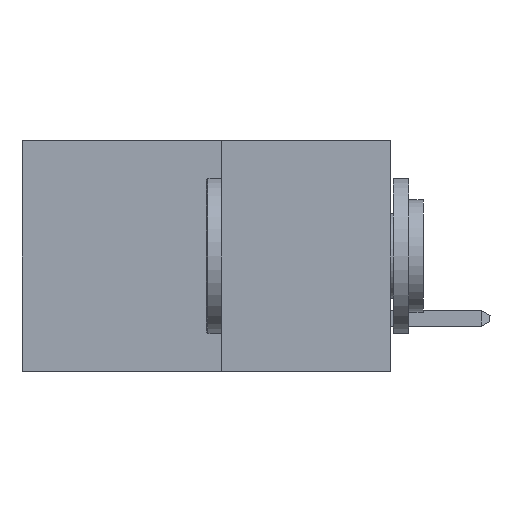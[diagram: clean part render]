
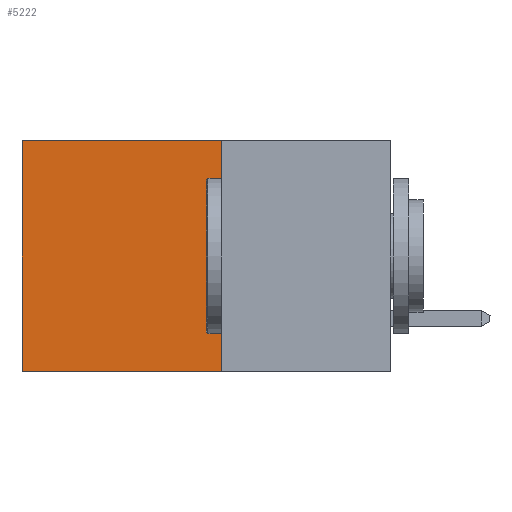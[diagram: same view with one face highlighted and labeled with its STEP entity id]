
A CAD part, left-side view. The second image highlights one B-rep face of the part: STEP entity #5222.
In plain terms, the highlighted planar face has unit normal (-1, 0, 0).
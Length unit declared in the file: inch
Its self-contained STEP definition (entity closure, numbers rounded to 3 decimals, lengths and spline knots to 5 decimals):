
#115 = ORIENTED_EDGE ( 'NONE', *, *, #12613, .F. ) ;
#355 = VERTEX_POINT ( 'NONE', #15876 ) ;
#586 = EDGE_CURVE ( 'NONE', #9196, #2411, #7843, .T. ) ;
#703 = VECTOR ( 'NONE', #13548, 39.37008 ) ;
#725 = CARTESIAN_POINT ( 'NONE',  ( 0.277, 0.27, -0.37 ) ) ;
#857 = DIRECTION ( 'NONE',  ( 0., 0., -1. ) ) ;
#893 = EDGE_CURVE ( 'NONE', #2411, #5199, #7447, .T. ) ;
#1137 = VECTOR ( 'NONE', #9937, 39.37008 ) ;
#1977 = LINE ( 'NONE', #725, #2400 ) ;
#2245 = FACE_OUTER_BOUND ( 'NONE', #8355, .T. ) ;
#2400 = VECTOR ( 'NONE', #857, 39.37008 ) ;
#2411 = VERTEX_POINT ( 'NONE', #9262 ) ;
#4274 = AXIS2_PLACEMENT_3D ( 'NONE', #14201, #14146, #14125 ) ;
#4590 = VECTOR ( 'NONE', #15267, 39.37008 ) ;
#5199 = VERTEX_POINT ( 'NONE', #14320 ) ;
#5222 = ADVANCED_FACE ( 'NONE', ( #2245 ), #14271, .F. ) ;
#6956 = EDGE_CURVE ( 'NONE', #9196, #355, #1977, .T. ) ;
#7447 = LINE ( 'NONE', #8086, #703 ) ;
#7487 = ORIENTED_EDGE ( 'NONE', *, *, #586, .T. ) ;
#7843 = LINE ( 'NONE', #13983, #1137 ) ;
#8086 = CARTESIAN_POINT ( 'NONE',  ( 0.277, 0.59, -0.37 ) ) ;
#8355 = EDGE_LOOP ( 'NONE', ( #14145, #115, #10643, #7487 ) ) ;
#9196 = VERTEX_POINT ( 'NONE', #12678 ) ;
#9262 = CARTESIAN_POINT ( 'NONE',  ( 0.277, 0.59, 0. ) ) ;
#9937 = DIRECTION ( 'NONE',  ( 0., 1., 0. ) ) ;
#10643 = ORIENTED_EDGE ( 'NONE', *, *, #6956, .F. ) ;
#12613 = EDGE_CURVE ( 'NONE', #355, #5199, #13869, .T. ) ;
#12678 = CARTESIAN_POINT ( 'NONE',  ( 0.277, 0.27, 0. ) ) ;
#12921 = CARTESIAN_POINT ( 'NONE',  ( 0.277, 0.27, -0.37 ) ) ;
#13548 = DIRECTION ( 'NONE',  ( 0., 0., -1. ) ) ;
#13869 = LINE ( 'NONE', #12921, #4590 ) ;
#13983 = CARTESIAN_POINT ( 'NONE',  ( 0.277, 0.27, 0. ) ) ;
#14125 = DIRECTION ( 'NONE',  ( 0., 0., -1. ) ) ;
#14145 = ORIENTED_EDGE ( 'NONE', *, *, #893, .T. ) ;
#14146 = DIRECTION ( 'NONE',  ( 1., 0., 0. ) ) ;
#14201 = CARTESIAN_POINT ( 'NONE',  ( 0.277, 0.27, -0.37 ) ) ;
#14271 = PLANE ( 'NONE',  #4274 ) ;
#14320 = CARTESIAN_POINT ( 'NONE',  ( 0.277, 0.59, -0.37 ) ) ;
#15267 = DIRECTION ( 'NONE',  ( 0., 1., 0. ) ) ;
#15876 = CARTESIAN_POINT ( 'NONE',  ( 0.277, 0.27, -0.37 ) ) ;
